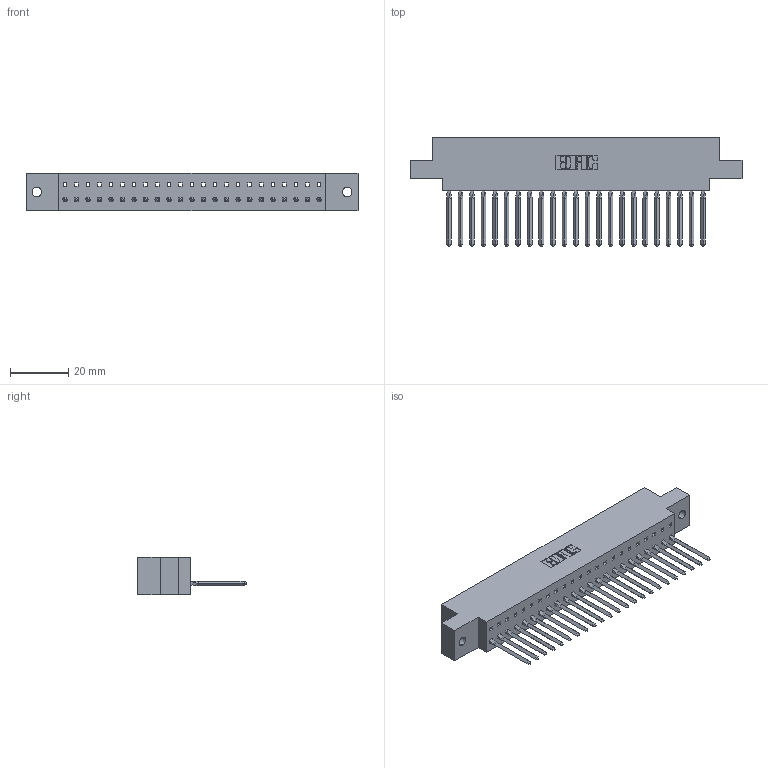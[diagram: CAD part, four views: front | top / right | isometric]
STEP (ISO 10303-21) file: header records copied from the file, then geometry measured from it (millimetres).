
FILE_DESCRIPTION (( 'STEP AP203' ), '1' );
FILE_NAME ('317-023-542-602.STEP', '2020-02-27T17:39:11', ( '' ), ( '' ), 'SwSTEP 2.0', 'SolidWorks 2016', '' );
FILE_SCHEMA (( 'CONFIG_CONTROL_DESIGN' ));
Length unit declared in the file: inch
Products named in the file (3): 317 Part_.144 Dia; 317-023-542-602; 317-290-003_542
Assembly tree (24 placements, depth 2):
  317-023-542-602
    317 Part_.144 Dia
    317-290-003_542  x23
Bounding box: 113.84 x 37.34 x 12.7 mm (x, y, z)
Volume: 17043.8 mm3; surface area: 20094.9 mm2
Topology: 24 solids, 24 shells, 1827 faces, 5266 edges, 3402 vertices
Faces by surface type: plane 1530, cylinder 205, bspline 92
Entity records: 34181 total; most frequent: CARTESIAN_POINT 6314, ORIENTED_EDGE 6000, DIRECTION 5034, EDGE_CURVE 3000, VECTOR 2830, LINE 2830, VERTEX_POINT 1994, AXIS2_PLACEMENT_3D 1102
